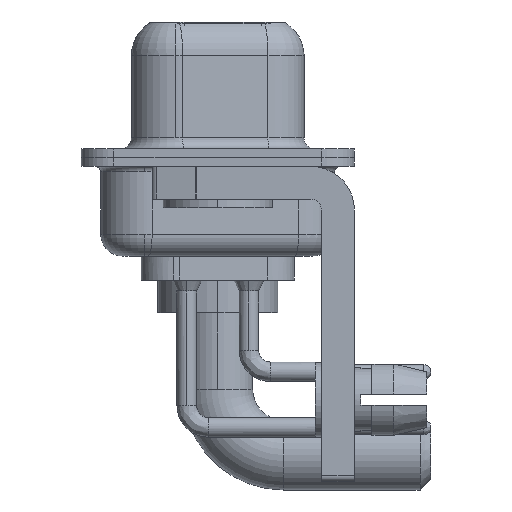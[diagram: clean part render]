
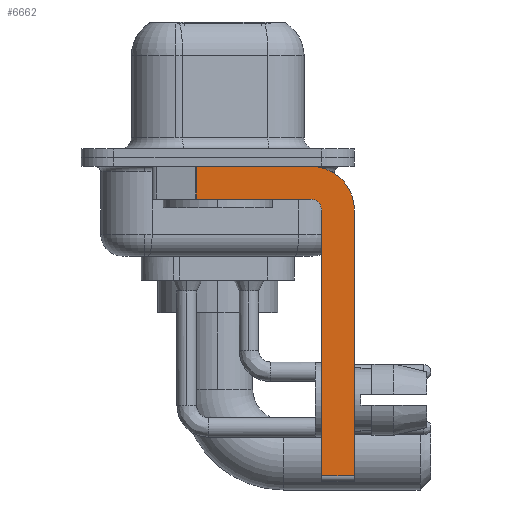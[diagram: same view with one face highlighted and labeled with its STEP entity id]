
A CAD part, left-side view. The second image highlights one B-rep face of the part: STEP entity #6662.
In plain terms, the highlighted planar face has unit normal (-1, 0, 0).
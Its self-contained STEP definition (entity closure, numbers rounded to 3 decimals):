
#148 = VECTOR ( 'NONE', #3389, 1000. ) ;
#191 = LINE ( 'NONE', #8512, #2196 ) ;
#220 = DIRECTION ( 'NONE',  ( -1., 0., 0. ) ) ;
#278 = DIRECTION ( 'NONE',  ( 0., 1., 0. ) ) ;
#326 = DIRECTION ( 'NONE',  ( 0., 0., -1. ) ) ;
#361 = EDGE_CURVE ( 'NONE', #7458, #5756, #6742, .T. ) ;
#543 = CARTESIAN_POINT ( 'NONE',  ( -2.9, -6.25, -14.55 ) ) ;
#583 = CARTESIAN_POINT ( 'NONE',  ( -2.9, -4.25, -2.4 ) ) ;
#1048 = EDGE_CURVE ( 'NONE', #7458, #2821, #1581, .T. ) ;
#1055 = FACE_OUTER_BOUND ( 'NONE', #12623, .T. ) ;
#1469 = VECTOR ( 'NONE', #2670, 1000. ) ;
#1581 = LINE ( 'NONE', #1876, #7130 ) ;
#1876 = CARTESIAN_POINT ( 'NONE',  ( -2.9, -4.25, -14.55 ) ) ;
#2196 = VECTOR ( 'NONE', #4207, 1000. ) ;
#2533 = AXIS2_PLACEMENT_3D ( 'NONE', #15429, #18187, #9495 ) ;
#2670 = DIRECTION ( 'NONE',  ( 0., 0., 1. ) ) ;
#2803 = ORIENTED_EDGE ( 'NONE', *, *, #1048, .T. ) ;
#2821 = VERTEX_POINT ( 'NONE', #543 ) ;
#3389 = DIRECTION ( 'NONE',  ( 0., 0., -1. ) ) ;
#3883 = CARTESIAN_POINT ( 'NONE',  ( -2.9, -4.75, -14.8 ) ) ;
#4018 = AXIS2_PLACEMENT_3D ( 'NONE', #7290, #220, #17346 ) ;
#4119 = EDGE_CURVE ( 'NONE', #10915, #6784, #6107, .T. ) ;
#4207 = DIRECTION ( 'NONE',  ( 0., 0., -1. ) ) ;
#4272 = ORIENTED_EDGE ( 'NONE', *, *, #361, .F. ) ;
#4677 = CARTESIAN_POINT ( 'NONE',  ( -2.9, 0.978, -0.4 ) ) ;
#5133 = CARTESIAN_POINT ( 'NONE',  ( -2.9, -4.75, -14.55 ) ) ;
#5199 = PLANE ( 'NONE',  #2533 ) ;
#5271 = EDGE_CURVE ( 'NONE', #13899, #15062, #15192, .T. ) ;
#5756 = VERTEX_POINT ( 'NONE', #17609 ) ;
#6107 = LINE ( 'NONE', #7355, #8309 ) ;
#6114 = CARTESIAN_POINT ( 'NONE',  ( -2.9, -4.25, -0.4 ) ) ;
#6412 = AXIS2_PLACEMENT_3D ( 'NONE', #583, #12131, #326 ) ;
#6662 = ADVANCED_FACE ( 'NONE', ( #1055 ), #5199, .F. ) ;
#6742 = LINE ( 'NONE', #3883, #1469 ) ;
#6784 = VERTEX_POINT ( 'NONE', #16952 ) ;
#6939 = ORIENTED_EDGE ( 'NONE', *, *, #4119, .F. ) ;
#7130 = VECTOR ( 'NONE', #13417, 1000. ) ;
#7286 = VERTEX_POINT ( 'NONE', #4677 ) ;
#7290 = CARTESIAN_POINT ( 'NONE',  ( -2.9, -4.25, -2.4 ) ) ;
#7355 = CARTESIAN_POINT ( 'NONE',  ( -2.9, -4.25, -1.9 ) ) ;
#7365 = LINE ( 'NONE', #13783, #16765 ) ;
#7458 = VERTEX_POINT ( 'NONE', #5133 ) ;
#8309 = VECTOR ( 'NONE', #278, 1000. ) ;
#8512 = CARTESIAN_POINT ( 'NONE',  ( -2.9, 0.978, -1.9 ) ) ;
#8845 = ORIENTED_EDGE ( 'NONE', *, *, #14862, .F. ) ;
#9214 = LINE ( 'NONE', #14771, #148 ) ;
#9495 = DIRECTION ( 'NONE',  ( 0., 0., -1. ) ) ;
#10915 = VERTEX_POINT ( 'NONE', #11793 ) ;
#11060 = DIRECTION ( 'NONE',  ( 0., -1., 0. ) ) ;
#11793 = CARTESIAN_POINT ( 'NONE',  ( -2.9, -4.25, -1.9 ) ) ;
#12131 = DIRECTION ( 'NONE',  ( 1., 0., 0. ) ) ;
#12623 = EDGE_LOOP ( 'NONE', ( #14059, #15633, #6939, #12764, #4272, #2803, #8845, #17735 ) ) ;
#12764 = ORIENTED_EDGE ( 'NONE', *, *, #14744, .F. ) ;
#13417 = DIRECTION ( 'NONE',  ( 0., -1., 0. ) ) ;
#13753 = EDGE_CURVE ( 'NONE', #7286, #6784, #191, .T. ) ;
#13783 = CARTESIAN_POINT ( 'NONE',  ( -2.9, 3., -0.4 ) ) ;
#13899 = VERTEX_POINT ( 'NONE', #6114 ) ;
#14059 = ORIENTED_EDGE ( 'NONE', *, *, #15205, .F. ) ;
#14624 = CIRCLE ( 'NONE', #4018, 0.5 ) ;
#14744 = EDGE_CURVE ( 'NONE', #5756, #10915, #14624, .T. ) ;
#14771 = CARTESIAN_POINT ( 'NONE',  ( -2.9, -6.25, -2.4 ) ) ;
#14862 = EDGE_CURVE ( 'NONE', #15062, #2821, #9214, .T. ) ;
#15062 = VERTEX_POINT ( 'NONE', #17225 ) ;
#15192 = CIRCLE ( 'NONE', #6412, 2. ) ;
#15205 = EDGE_CURVE ( 'NONE', #7286, #13899, #7365, .T. ) ;
#15429 = CARTESIAN_POINT ( 'NONE',  ( -2.9, -4.25, -2.4 ) ) ;
#15633 = ORIENTED_EDGE ( 'NONE', *, *, #13753, .T. ) ;
#16765 = VECTOR ( 'NONE', #11060, 1000. ) ;
#16952 = CARTESIAN_POINT ( 'NONE',  ( -2.9, 0.978, -1.9 ) ) ;
#17225 = CARTESIAN_POINT ( 'NONE',  ( -2.9, -6.25, -2.4 ) ) ;
#17346 = DIRECTION ( 'NONE',  ( 0., 0., 1. ) ) ;
#17609 = CARTESIAN_POINT ( 'NONE',  ( -2.9, -4.75, -2.4 ) ) ;
#17735 = ORIENTED_EDGE ( 'NONE', *, *, #5271, .F. ) ;
#18187 = DIRECTION ( 'NONE',  ( 1., 0., 0. ) ) ;
